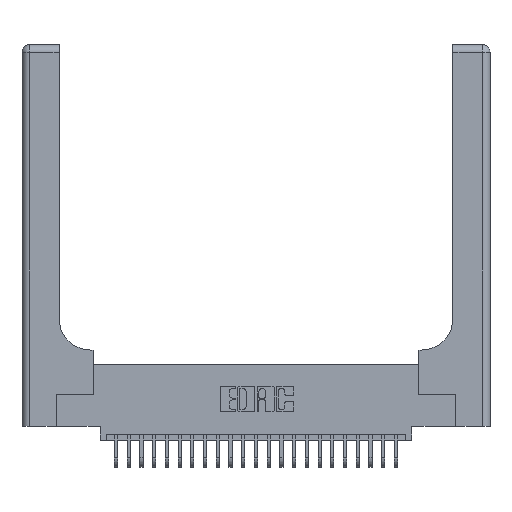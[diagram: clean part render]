
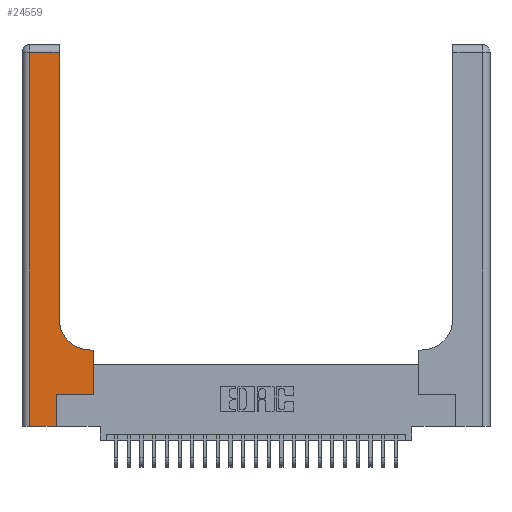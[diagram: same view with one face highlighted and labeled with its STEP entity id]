
A CAD part, top view. The second image highlights one B-rep face of the part: STEP entity #24559.
In plain terms, the highlighted planar face has unit normal (0, 0, 1).
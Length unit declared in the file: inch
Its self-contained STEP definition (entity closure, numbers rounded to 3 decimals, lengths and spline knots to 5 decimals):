
#86 = VERTEX_POINT ( 'NONE', #19109 ) ;
#1019 = ORIENTED_EDGE ( 'NONE', *, *, #19255, .T. ) ;
#1105 = ORIENTED_EDGE ( 'NONE', *, *, #3666, .T. ) ;
#1600 = VERTEX_POINT ( 'NONE', #4267 ) ;
#2520 = EDGE_CURVE ( 'NONE', #14111, #86, #14777, .T. ) ;
#3268 = DIRECTION ( 'NONE',  ( 0., 0., -1. ) ) ;
#3483 = EDGE_LOOP ( 'NONE', ( #3659, #17941, #5392, #13416, #8783, #1019, #1105, #13412, #20590 ) ) ;
#3659 = ORIENTED_EDGE ( 'NONE', *, *, #2520, .T. ) ;
#3666 = EDGE_CURVE ( 'NONE', #12155, #17946, #17374, .T. ) ;
#4267 = CARTESIAN_POINT ( 'NONE',  ( 0.269, 0.25, 0.37 ) ) ;
#4448 = CARTESIAN_POINT ( 'NONE',  ( 0.2915, 0.6, 0.37 ) ) ;
#4518 = EDGE_CURVE ( 'NONE', #86, #20583, #7378, .T. ) ;
#4716 = CARTESIAN_POINT ( 'NONE',  ( 0.2915, 0.85, 0.37 ) ) ;
#4814 = DIRECTION ( 'NONE',  ( 0., 0., -1. ) ) ;
#4984 = CARTESIAN_POINT ( 'NONE',  ( 0.269, 0., 0.37 ) ) ;
#5392 = ORIENTED_EDGE ( 'NONE', *, *, #22050, .T. ) ;
#6083 = VECTOR ( 'NONE', #7396, 39.37008 ) ;
#7298 = CARTESIAN_POINT ( 'NONE',  ( 0.5585, 0.25, 0.37 ) ) ;
#7378 = LINE ( 'NONE', #20694, #26323 ) ;
#7396 = DIRECTION ( 'NONE',  ( 0., 1., 0. ) ) ;
#7653 = LINE ( 'NONE', #4448, #23548 ) ;
#7739 = VERTEX_POINT ( 'NONE', #17428 ) ;
#8783 = ORIENTED_EDGE ( 'NONE', *, *, #10040, .T. ) ;
#9331 = CIRCLE ( 'NONE', #15911, 0.25 ) ;
#9998 = PLANE ( 'NONE',  #12750 ) ;
#10040 = EDGE_CURVE ( 'NONE', #11314, #1600, #21576, .T. ) ;
#10155 = DIRECTION ( 'NONE',  ( -1., 0., 0. ) ) ;
#10372 = EDGE_CURVE ( 'NONE', #11726, #14111, #9331, .T. ) ;
#11314 = VERTEX_POINT ( 'NONE', #4984 ) ;
#11660 = CARTESIAN_POINT ( 'NONE',  ( 0.269, 0.25, 0.37 ) ) ;
#11671 = CARTESIAN_POINT ( 'NONE',  ( 0.2915, 3., 0.37 ) ) ;
#11726 = VERTEX_POINT ( 'NONE', #26059 ) ;
#11917 = LINE ( 'NONE', #15957, #27530 ) ;
#12051 = CARTESIAN_POINT ( 'NONE',  ( 0., 3., 0.37 ) ) ;
#12155 = VERTEX_POINT ( 'NONE', #26069 ) ;
#12750 = AXIS2_PLACEMENT_3D ( 'NONE', #12051, #3268, #20190 ) ;
#12756 = EDGE_CURVE ( 'NONE', #7739, #11314, #11917, .T. ) ;
#13412 = ORIENTED_EDGE ( 'NONE', *, *, #19020, .T. ) ;
#13416 = ORIENTED_EDGE ( 'NONE', *, *, #12756, .T. ) ;
#13662 = VECTOR ( 'NONE', #16356, 39.37008 ) ;
#14111 = VERTEX_POINT ( 'NONE', #4716 ) ;
#14777 = LINE ( 'NONE', #11671, #20121 ) ;
#15911 = AXIS2_PLACEMENT_3D ( 'NONE', #19409, #4814, #19602 ) ;
#15957 = CARTESIAN_POINT ( 'NONE',  ( 0., 0., 0.37 ) ) ;
#16356 = DIRECTION ( 'NONE',  ( 0., 1., 0. ) ) ;
#17374 = LINE ( 'NONE', #7298, #6083 ) ;
#17428 = CARTESIAN_POINT ( 'NONE',  ( 0.06, 0., 0.37 ) ) ;
#17941 = ORIENTED_EDGE ( 'NONE', *, *, #4518, .T. ) ;
#17946 = VERTEX_POINT ( 'NONE', #24882 ) ;
#19020 = EDGE_CURVE ( 'NONE', #17946, #11726, #7653, .T. ) ;
#19109 = CARTESIAN_POINT ( 'NONE',  ( 0.2915, 2.94, 0.37 ) ) ;
#19255 = EDGE_CURVE ( 'NONE', #1600, #12155, #25873, .T. ) ;
#19409 = CARTESIAN_POINT ( 'NONE',  ( 0.5415, 0.85, 0.37 ) ) ;
#19602 = DIRECTION ( 'NONE',  ( 1., 0., 0. ) ) ;
#19806 = DIRECTION ( 'NONE',  ( 0., 1., 0. ) ) ;
#20086 = LINE ( 'NONE', #20096, #25774 ) ;
#20096 = CARTESIAN_POINT ( 'NONE',  ( 0.06, 3., 0.37 ) ) ;
#20121 = VECTOR ( 'NONE', #19806, 39.37008 ) ;
#20190 = DIRECTION ( 'NONE',  ( -1., 0., 0. ) ) ;
#20451 = DIRECTION ( 'NONE',  ( 1., 0., 0. ) ) ;
#20583 = VERTEX_POINT ( 'NONE', #27398 ) ;
#20590 = ORIENTED_EDGE ( 'NONE', *, *, #10372, .T. ) ;
#20694 = CARTESIAN_POINT ( 'NONE',  ( 0., 2.94, 0.37 ) ) ;
#21576 = LINE ( 'NONE', #22668, #13662 ) ;
#22050 = EDGE_CURVE ( 'NONE', #20583, #7739, #20086, .T. ) ;
#22668 = CARTESIAN_POINT ( 'NONE',  ( 0.269, 0., 0.37 ) ) ;
#23548 = VECTOR ( 'NONE', #23673, 39.37008 ) ;
#23673 = DIRECTION ( 'NONE',  ( -1., 0., 0. ) ) ;
#24108 = DIRECTION ( 'NONE',  ( 1., 0., 0. ) ) ;
#24559 = ADVANCED_FACE ( 'NONE', ( #25304 ), #9998, .F. ) ;
#24882 = CARTESIAN_POINT ( 'NONE',  ( 0.5585, 0.6, 0.37 ) ) ;
#25304 = FACE_OUTER_BOUND ( 'NONE', #3483, .T. ) ;
#25774 = VECTOR ( 'NONE', #26246, 39.37008 ) ;
#25873 = LINE ( 'NONE', #11660, #27259 ) ;
#26059 = CARTESIAN_POINT ( 'NONE',  ( 0.5415, 0.6, 0.37 ) ) ;
#26069 = CARTESIAN_POINT ( 'NONE',  ( 0.5585, 0.25, 0.37 ) ) ;
#26246 = DIRECTION ( 'NONE',  ( 0., -1., 0. ) ) ;
#26323 = VECTOR ( 'NONE', #10155, 39.37008 ) ;
#27259 = VECTOR ( 'NONE', #20451, 39.37008 ) ;
#27398 = CARTESIAN_POINT ( 'NONE',  ( 0.06, 2.94, 0.37 ) ) ;
#27530 = VECTOR ( 'NONE', #24108, 39.37008 ) ;
